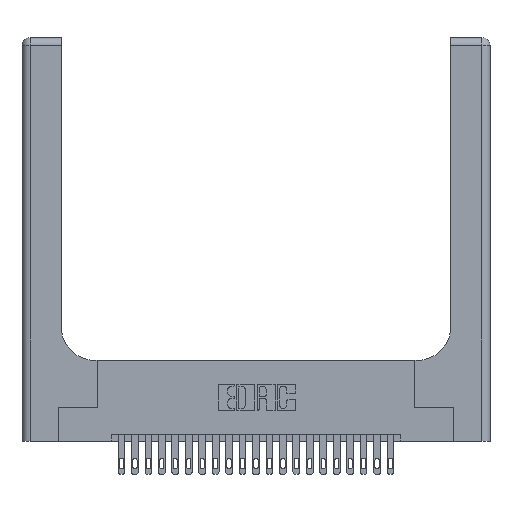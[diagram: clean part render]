
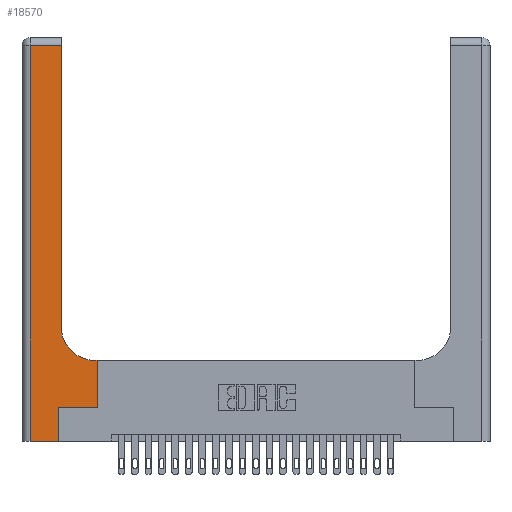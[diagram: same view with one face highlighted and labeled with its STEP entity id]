
A CAD part, top view. The second image highlights one B-rep face of the part: STEP entity #18570.
In plain terms, the highlighted planar face has unit normal (0, 0, 1).
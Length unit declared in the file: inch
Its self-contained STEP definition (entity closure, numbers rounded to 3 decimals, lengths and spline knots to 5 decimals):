
#604 = ORIENTED_EDGE ( 'NONE', *, *, #10300, .T. ) ;
#818 = CARTESIAN_POINT ( 'NONE',  ( 0.5415, 0.6, 0.37 ) ) ;
#896 = DIRECTION ( 'NONE',  ( 0., 1., 0. ) ) ;
#1540 = CARTESIAN_POINT ( 'NONE',  ( 0.269, 0.25, 0.37 ) ) ;
#2191 = VECTOR ( 'NONE', #19603, 39.37008 ) ;
#2236 = VERTEX_POINT ( 'NONE', #7997 ) ;
#2408 = EDGE_CURVE ( 'NONE', #8542, #13586, #9516, .T. ) ;
#2642 = LINE ( 'NONE', #11930, #17053 ) ;
#3176 = CARTESIAN_POINT ( 'NONE',  ( 0., 3., 0.37 ) ) ;
#3455 = ORIENTED_EDGE ( 'NONE', *, *, #20810, .T. ) ;
#4292 = VERTEX_POINT ( 'NONE', #7536 ) ;
#4768 = DIRECTION ( 'NONE',  ( 1., 0., 0. ) ) ;
#4968 = DIRECTION ( 'NONE',  ( -1., 0., 0. ) ) ;
#5743 = EDGE_CURVE ( 'NONE', #11103, #9917, #21460, .T. ) ;
#6712 = LINE ( 'NONE', #15488, #12599 ) ;
#7007 = ORIENTED_EDGE ( 'NONE', *, *, #13508, .T. ) ;
#7536 = CARTESIAN_POINT ( 'NONE',  ( 0.06, 2.94, 0.37 ) ) ;
#7771 = CIRCLE ( 'NONE', #14482, 0.25 ) ;
#7861 = DIRECTION ( 'NONE',  ( -1., 0., 0. ) ) ;
#7933 = VECTOR ( 'NONE', #4968, 39.37008 ) ;
#7997 = CARTESIAN_POINT ( 'NONE',  ( 0.06, 0., 0.37 ) ) ;
#8044 = VECTOR ( 'NONE', #7861, 39.37008 ) ;
#8157 = LINE ( 'NONE', #21585, #19353 ) ;
#8160 = CARTESIAN_POINT ( 'NONE',  ( 0.06, 3., 0.37 ) ) ;
#8490 = VERTEX_POINT ( 'NONE', #1540 ) ;
#8542 = VERTEX_POINT ( 'NONE', #20380 ) ;
#8653 = DIRECTION ( 'NONE',  ( 0., 0., -1. ) ) ;
#8813 = CARTESIAN_POINT ( 'NONE',  ( 0.2915, 3., 0.37 ) ) ;
#9516 = LINE ( 'NONE', #17674, #2191 ) ;
#9584 = EDGE_CURVE ( 'NONE', #2236, #18280, #2642, .T. ) ;
#9917 = VERTEX_POINT ( 'NONE', #22785 ) ;
#10300 = EDGE_CURVE ( 'NONE', #18280, #8490, #8157, .T. ) ;
#10685 = LINE ( 'NONE', #13090, #8044 ) ;
#10972 = ORIENTED_EDGE ( 'NONE', *, *, #16834, .T. ) ;
#11103 = VERTEX_POINT ( 'NONE', #11710 ) ;
#11187 = VECTOR ( 'NONE', #13941, 39.37008 ) ;
#11292 = DIRECTION ( 'NONE',  ( 0., 1., 0. ) ) ;
#11710 = CARTESIAN_POINT ( 'NONE',  ( 0.2915, 0.85, 0.37 ) ) ;
#11830 = ORIENTED_EDGE ( 'NONE', *, *, #16648, .T. ) ;
#11930 = CARTESIAN_POINT ( 'NONE',  ( 0., 0., 0.37 ) ) ;
#12273 = FACE_OUTER_BOUND ( 'NONE', #15056, .T. ) ;
#12546 = PLANE ( 'NONE',  #13428 ) ;
#12553 = DIRECTION ( 'NONE',  ( 0., 0., -1. ) ) ;
#12599 = VECTOR ( 'NONE', #21174, 39.37008 ) ;
#13090 = CARTESIAN_POINT ( 'NONE',  ( 0., 2.94, 0.37 ) ) ;
#13428 = AXIS2_PLACEMENT_3D ( 'NONE', #3176, #8653, #14595 ) ;
#13508 = EDGE_CURVE ( 'NONE', #9917, #4292, #10685, .T. ) ;
#13586 = VERTEX_POINT ( 'NONE', #14534 ) ;
#13941 = DIRECTION ( 'NONE',  ( 0., -1., 0. ) ) ;
#14482 = AXIS2_PLACEMENT_3D ( 'NONE', #23712, #12553, #21886 ) ;
#14534 = CARTESIAN_POINT ( 'NONE',  ( 0.5585, 0.6, 0.37 ) ) ;
#14595 = DIRECTION ( 'NONE',  ( -1., 0., 0. ) ) ;
#14954 = CARTESIAN_POINT ( 'NONE',  ( 0.269, 0., 0.37 ) ) ;
#14985 = VECTOR ( 'NONE', #11292, 39.37008 ) ;
#15056 = EDGE_LOOP ( 'NONE', ( #17302, #7007, #11830, #15591, #604, #21772, #19899, #10972, #3455 ) ) ;
#15488 = CARTESIAN_POINT ( 'NONE',  ( 0.269, 0.25, 0.37 ) ) ;
#15591 = ORIENTED_EDGE ( 'NONE', *, *, #9584, .T. ) ;
#16648 = EDGE_CURVE ( 'NONE', #4292, #2236, #21822, .T. ) ;
#16834 = EDGE_CURVE ( 'NONE', #13586, #17226, #24208, .T. ) ;
#17053 = VECTOR ( 'NONE', #4768, 39.37008 ) ;
#17226 = VERTEX_POINT ( 'NONE', #818 ) ;
#17302 = ORIENTED_EDGE ( 'NONE', *, *, #5743, .T. ) ;
#17674 = CARTESIAN_POINT ( 'NONE',  ( 0.5585, 0.25, 0.37 ) ) ;
#18280 = VERTEX_POINT ( 'NONE', #14954 ) ;
#18570 = ADVANCED_FACE ( 'NONE', ( #12273 ), #12546, .F. ) ;
#19353 = VECTOR ( 'NONE', #896, 39.37008 ) ;
#19603 = DIRECTION ( 'NONE',  ( 0., 1., 0. ) ) ;
#19899 = ORIENTED_EDGE ( 'NONE', *, *, #2408, .T. ) ;
#20380 = CARTESIAN_POINT ( 'NONE',  ( 0.5585, 0.25, 0.37 ) ) ;
#20810 = EDGE_CURVE ( 'NONE', #17226, #11103, #7771, .T. ) ;
#21174 = DIRECTION ( 'NONE',  ( 1., 0., 0. ) ) ;
#21460 = LINE ( 'NONE', #8813, #14985 ) ;
#21585 = CARTESIAN_POINT ( 'NONE',  ( 0.269, 0., 0.37 ) ) ;
#21772 = ORIENTED_EDGE ( 'NONE', *, *, #24166, .T. ) ;
#21822 = LINE ( 'NONE', #8160, #11187 ) ;
#21886 = DIRECTION ( 'NONE',  ( 1., 0., 0. ) ) ;
#22785 = CARTESIAN_POINT ( 'NONE',  ( 0.2915, 2.94, 0.37 ) ) ;
#23712 = CARTESIAN_POINT ( 'NONE',  ( 0.5415, 0.85, 0.37 ) ) ;
#23943 = CARTESIAN_POINT ( 'NONE',  ( 0.2915, 0.6, 0.37 ) ) ;
#24166 = EDGE_CURVE ( 'NONE', #8490, #8542, #6712, .T. ) ;
#24208 = LINE ( 'NONE', #23943, #7933 ) ;
